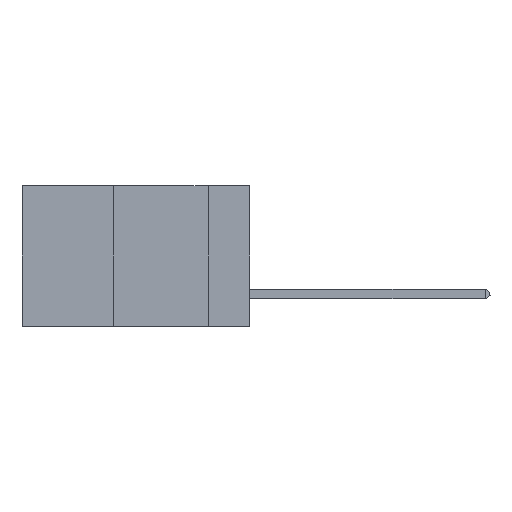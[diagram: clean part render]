
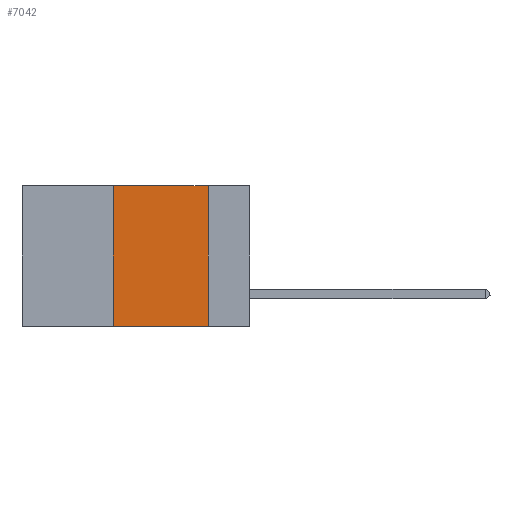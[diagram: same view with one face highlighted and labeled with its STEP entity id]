
A CAD part, left-side view. The second image highlights one B-rep face of the part: STEP entity #7042.
In plain terms, the highlighted planar face has unit normal (-1, 0, 0).
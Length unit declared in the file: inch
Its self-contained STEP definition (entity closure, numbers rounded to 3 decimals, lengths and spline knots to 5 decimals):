
#388 = CARTESIAN_POINT ( 'NONE',  ( 0., 0.11, 0. ) ) ;
#891 = PLANE ( 'NONE',  #8659 ) ;
#1228 = LINE ( 'NONE', #31791, #31872 ) ;
#1938 = CARTESIAN_POINT ( 'NONE',  ( 0., 0.36, -0.37 ) ) ;
#3454 = VECTOR ( 'NONE', #30799, 39.37008 ) ;
#3469 = CARTESIAN_POINT ( 'NONE',  ( 0., 0.11, -0.37 ) ) ;
#3820 = DIRECTION ( 'NONE',  ( 0., 0., -1. ) ) ;
#4510 = VERTEX_POINT ( 'NONE', #26560 ) ;
#5820 = ORIENTED_EDGE ( 'NONE', *, *, #15735, .T. ) ;
#7042 = ADVANCED_FACE ( 'NONE', ( #27784 ), #891, .F. ) ;
#7795 = VERTEX_POINT ( 'NONE', #388 ) ;
#8215 = ORIENTED_EDGE ( 'NONE', *, *, #22436, .F. ) ;
#8659 = AXIS2_PLACEMENT_3D ( 'NONE', #23817, #31601, #16311 ) ;
#11151 = CARTESIAN_POINT ( 'NONE',  ( 0., 0.11, 0. ) ) ;
#11216 = VERTEX_POINT ( 'NONE', #3469 ) ;
#11515 = ORIENTED_EDGE ( 'NONE', *, *, #26036, .F. ) ;
#12752 = CARTESIAN_POINT ( 'NONE',  ( 0., 0.36, 0. ) ) ;
#14951 = LINE ( 'NONE', #12752, #3454 ) ;
#14953 = VECTOR ( 'NONE', #27668, 39.37008 ) ;
#15735 = EDGE_CURVE ( 'NONE', #30247, #11216, #1228, .T. ) ;
#15961 = ORIENTED_EDGE ( 'NONE', *, *, #24485, .F. ) ;
#16311 = DIRECTION ( 'NONE',  ( 0., 0., -1. ) ) ;
#16503 = DIRECTION ( 'NONE',  ( 0., -1., 0. ) ) ;
#17238 = CARTESIAN_POINT ( 'NONE',  ( 0., 0.6, 0. ) ) ;
#19506 = LINE ( 'NONE', #11151, #22320 ) ;
#22320 = VECTOR ( 'NONE', #3820, 39.37008 ) ;
#22436 = EDGE_CURVE ( 'NONE', #7795, #11216, #19506, .T. ) ;
#23817 = CARTESIAN_POINT ( 'NONE',  ( 0., 0.6, 0. ) ) ;
#24485 = EDGE_CURVE ( 'NONE', #4510, #7795, #30536, .T. ) ;
#26036 = EDGE_CURVE ( 'NONE', #30247, #4510, #14951, .T. ) ;
#26560 = CARTESIAN_POINT ( 'NONE',  ( 0., 0.36, 0. ) ) ;
#27668 = DIRECTION ( 'NONE',  ( 0., -1., 0. ) ) ;
#27784 = FACE_OUTER_BOUND ( 'NONE', #32565, .T. ) ;
#30247 = VERTEX_POINT ( 'NONE', #1938 ) ;
#30536 = LINE ( 'NONE', #17238, #14953 ) ;
#30799 = DIRECTION ( 'NONE',  ( 0., 0., 1. ) ) ;
#31601 = DIRECTION ( 'NONE',  ( 1., 0., 0. ) ) ;
#31791 = CARTESIAN_POINT ( 'NONE',  ( 0., 0.6, -0.37 ) ) ;
#31872 = VECTOR ( 'NONE', #16503, 39.37008 ) ;
#32565 = EDGE_LOOP ( 'NONE', ( #8215, #15961, #11515, #5820 ) ) ;
